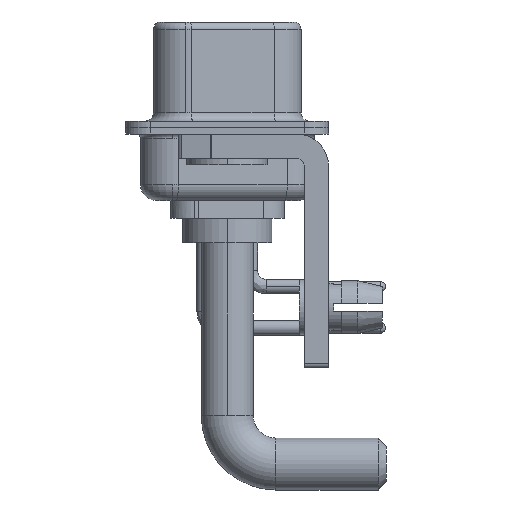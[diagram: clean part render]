
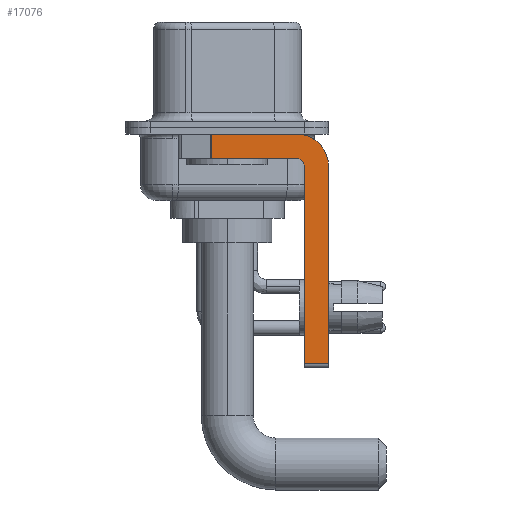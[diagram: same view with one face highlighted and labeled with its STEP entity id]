
A CAD part, left-side view. The second image highlights one B-rep face of the part: STEP entity #17076.
In plain terms, the highlighted planar face has unit normal (-1, 0, 0).
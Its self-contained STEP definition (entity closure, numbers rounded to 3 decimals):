
#12 = EDGE_LOOP ( 'NONE', ( #10016, #23149, #15559, #20365, #10614, #5583, #3075, #23821 ) ) ;
#63 = VERTEX_POINT ( 'NONE', #6994 ) ;
#229 = AXIS2_PLACEMENT_3D ( 'NONE', #13372, #20791, #23031 ) ;
#1329 = LINE ( 'NONE', #24331, #3808 ) ;
#1341 = EDGE_CURVE ( 'NONE', #10664, #5473, #8232, .T. ) ;
#1461 = CIRCLE ( 'NONE', #3492, 0.5 ) ;
#1505 = CARTESIAN_POINT ( 'NONE',  ( -2.9, -4.25, -2.4 ) ) ;
#1706 = VERTEX_POINT ( 'NONE', #12320 ) ;
#1727 = VERTEX_POINT ( 'NONE', #18254 ) ;
#3075 = ORIENTED_EDGE ( 'NONE', *, *, #12843, .F. ) ;
#3492 = AXIS2_PLACEMENT_3D ( 'NONE', #10282, #16209, #18343 ) ;
#3723 = LINE ( 'NONE', #10991, #11971 ) ;
#3808 = VECTOR ( 'NONE', #7130, 1000. ) ;
#4957 = VERTEX_POINT ( 'NONE', #5643 ) ;
#5353 = DIRECTION ( 'NONE',  ( 0., -1., 0. ) ) ;
#5473 = VERTEX_POINT ( 'NONE', #11746 ) ;
#5583 = ORIENTED_EDGE ( 'NONE', *, *, #15238, .T. ) ;
#5643 = CARTESIAN_POINT ( 'NONE',  ( -2.9, 0.978, -1.9 ) ) ;
#5709 = PLANE ( 'NONE',  #229 ) ;
#6170 = EDGE_CURVE ( 'NONE', #10581, #4957, #9329, .T. ) ;
#6635 = EDGE_CURVE ( 'NONE', #10581, #10664, #3723, .T. ) ;
#6786 = CARTESIAN_POINT ( 'NONE',  ( -2.9, 0.978, -0.4 ) ) ;
#6994 = CARTESIAN_POINT ( 'NONE',  ( -2.9, -4.75, -2.4 ) ) ;
#7130 = DIRECTION ( 'NONE',  ( 0., -1., 0. ) ) ;
#7569 = VECTOR ( 'NONE', #15113, 1000. ) ;
#7788 = VERTEX_POINT ( 'NONE', #16432 ) ;
#8232 = CIRCLE ( 'NONE', #14663, 2. ) ;
#8568 = LINE ( 'NONE', #8825, #22170 ) ;
#8825 = CARTESIAN_POINT ( 'NONE',  ( -2.9, -6.25, -2.4 ) ) ;
#9113 = LINE ( 'NONE', #19027, #13414 ) ;
#9329 = LINE ( 'NONE', #18508, #7569 ) ;
#10016 = ORIENTED_EDGE ( 'NONE', *, *, #6635, .F. ) ;
#10282 = CARTESIAN_POINT ( 'NONE',  ( -2.9, -4.25, -2.4 ) ) ;
#10445 = EDGE_CURVE ( 'NONE', #63, #1706, #1461, .T. ) ;
#10473 = CARTESIAN_POINT ( 'NONE',  ( -2.9, -4.75, -14.8 ) ) ;
#10555 = DIRECTION ( 'NONE',  ( 0., 0., -1. ) ) ;
#10581 = VERTEX_POINT ( 'NONE', #6786 ) ;
#10614 = ORIENTED_EDGE ( 'NONE', *, *, #14316, .F. ) ;
#10664 = VERTEX_POINT ( 'NONE', #12931 ) ;
#10724 = DIRECTION ( 'NONE',  ( 0., 0., 1. ) ) ;
#10991 = CARTESIAN_POINT ( 'NONE',  ( -2.9, 3., -0.4 ) ) ;
#11746 = CARTESIAN_POINT ( 'NONE',  ( -2.9, -6.25, -2.4 ) ) ;
#11971 = VECTOR ( 'NONE', #5353, 1000. ) ;
#12320 = CARTESIAN_POINT ( 'NONE',  ( -2.9, -4.25, -1.9 ) ) ;
#12843 = EDGE_CURVE ( 'NONE', #5473, #1727, #8568, .T. ) ;
#12871 = DIRECTION ( 'NONE',  ( 0., 1., 0. ) ) ;
#12931 = CARTESIAN_POINT ( 'NONE',  ( -2.9, -4.25, -0.4 ) ) ;
#12959 = DIRECTION ( 'NONE',  ( 0., 0., -1. ) ) ;
#13372 = CARTESIAN_POINT ( 'NONE',  ( -2.9, -4.25, -2.4 ) ) ;
#13414 = VECTOR ( 'NONE', #12871, 1000. ) ;
#14133 = LINE ( 'NONE', #10473, #24219 ) ;
#14316 = EDGE_CURVE ( 'NONE', #7788, #63, #14133, .T. ) ;
#14663 = AXIS2_PLACEMENT_3D ( 'NONE', #1505, #18994, #12959 ) ;
#15113 = DIRECTION ( 'NONE',  ( 0., 0., -1. ) ) ;
#15238 = EDGE_CURVE ( 'NONE', #7788, #1727, #1329, .T. ) ;
#15559 = ORIENTED_EDGE ( 'NONE', *, *, #15799, .F. ) ;
#15799 = EDGE_CURVE ( 'NONE', #1706, #4957, #9113, .T. ) ;
#16209 = DIRECTION ( 'NONE',  ( -1., 0., 0. ) ) ;
#16432 = CARTESIAN_POINT ( 'NONE',  ( -2.9, -4.75, -14.55 ) ) ;
#17076 = ADVANCED_FACE ( 'NONE', ( #22913 ), #5709, .F. ) ;
#18254 = CARTESIAN_POINT ( 'NONE',  ( -2.9, -6.25, -14.55 ) ) ;
#18343 = DIRECTION ( 'NONE',  ( 0., 0., 1. ) ) ;
#18508 = CARTESIAN_POINT ( 'NONE',  ( -2.9, 0.978, -1.9 ) ) ;
#18994 = DIRECTION ( 'NONE',  ( 1., 0., 0. ) ) ;
#19027 = CARTESIAN_POINT ( 'NONE',  ( -2.9, -4.25, -1.9 ) ) ;
#20365 = ORIENTED_EDGE ( 'NONE', *, *, #10445, .F. ) ;
#20791 = DIRECTION ( 'NONE',  ( 1., 0., 0. ) ) ;
#22170 = VECTOR ( 'NONE', #10555, 1000. ) ;
#22913 = FACE_OUTER_BOUND ( 'NONE', #12, .T. ) ;
#23031 = DIRECTION ( 'NONE',  ( 0., 0., -1. ) ) ;
#23149 = ORIENTED_EDGE ( 'NONE', *, *, #6170, .T. ) ;
#23821 = ORIENTED_EDGE ( 'NONE', *, *, #1341, .F. ) ;
#24219 = VECTOR ( 'NONE', #10724, 1000. ) ;
#24331 = CARTESIAN_POINT ( 'NONE',  ( -2.9, -4.25, -14.55 ) ) ;
